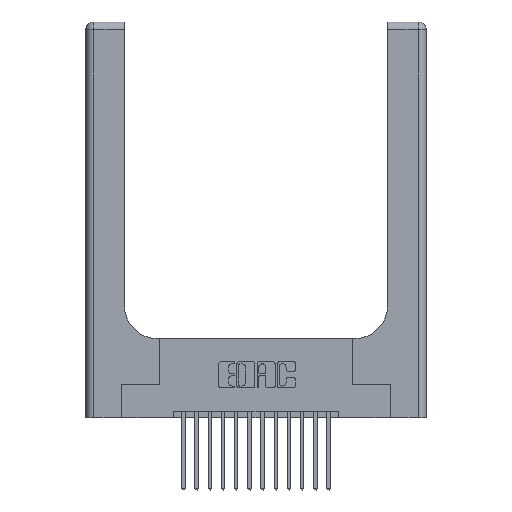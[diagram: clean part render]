
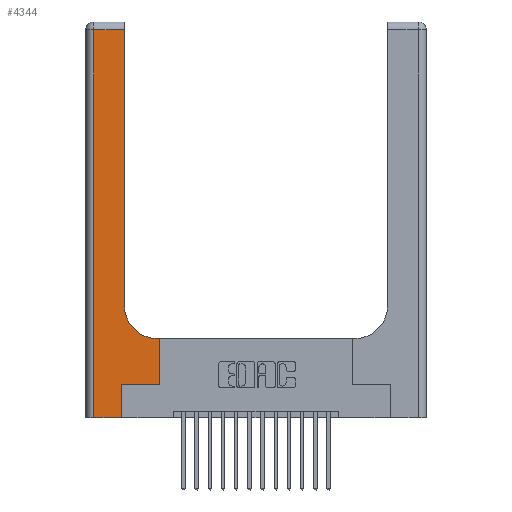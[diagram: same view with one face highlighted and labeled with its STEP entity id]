
A CAD part, top view. The second image highlights one B-rep face of the part: STEP entity #4344.
In plain terms, the highlighted planar face has unit normal (0, 0, 1).
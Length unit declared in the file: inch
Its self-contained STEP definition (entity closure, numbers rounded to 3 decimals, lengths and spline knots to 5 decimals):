
#13 = VECTOR ( 'NONE', #11765, 39.37008 ) ;
#380 = VECTOR ( 'NONE', #10703, 39.37008 ) ;
#407 = AXIS2_PLACEMENT_3D ( 'NONE', #4838, #15004, #6327 ) ;
#597 = LINE ( 'NONE', #6414, #7862 ) ;
#671 = LINE ( 'NONE', #1080, #4039 ) ;
#938 = VECTOR ( 'NONE', #16329, 39.37008 ) ;
#1080 = CARTESIAN_POINT ( 'NONE',  ( 0.269, 0.25, 0.37 ) ) ;
#1119 = CARTESIAN_POINT ( 'NONE',  ( 0.2915, 0.85, 0.37 ) ) ;
#1162 = ORIENTED_EDGE ( 'NONE', *, *, #1350, .T. ) ;
#1229 = VERTEX_POINT ( 'NONE', #1533 ) ;
#1254 = ORIENTED_EDGE ( 'NONE', *, *, #16557, .T. ) ;
#1350 = EDGE_CURVE ( 'NONE', #1229, #7404, #18650, .T. ) ;
#1461 = DIRECTION ( 'NONE',  ( -1., 0., 0. ) ) ;
#1533 = CARTESIAN_POINT ( 'NONE',  ( 0.5415, 0.6, 0.37 ) ) ;
#2022 = EDGE_CURVE ( 'NONE', #10979, #4656, #597, .T. ) ;
#2251 = VECTOR ( 'NONE', #11056, 39.37008 ) ;
#2411 = CARTESIAN_POINT ( 'NONE',  ( 0.06, 2.94, 0.37 ) ) ;
#2652 = AXIS2_PLACEMENT_3D ( 'NONE', #6569, #6552, #6879 ) ;
#2978 = EDGE_LOOP ( 'NONE', ( #9357, #15954, #17317, #1254, #3291, #14676, #6632, #12477, #1162 ) ) ;
#3042 = CARTESIAN_POINT ( 'NONE',  ( 0., 0., 0.37 ) ) ;
#3291 = ORIENTED_EDGE ( 'NONE', *, *, #2022, .T. ) ;
#3384 = LINE ( 'NONE', #3042, #13 ) ;
#3390 = PLANE ( 'NONE',  #407 ) ;
#4039 = VECTOR ( 'NONE', #11238, 39.37008 ) ;
#4344 = ADVANCED_FACE ( 'NONE', ( #7776 ), #3390, .F. ) ;
#4435 = LINE ( 'NONE', #15876, #15110 ) ;
#4656 = VERTEX_POINT ( 'NONE', #17050 ) ;
#4753 = LINE ( 'NONE', #6211, #938 ) ;
#4784 = EDGE_CURVE ( 'NONE', #7404, #6162, #4753, .T. ) ;
#4836 = CARTESIAN_POINT ( 'NONE',  ( 0.5585, 0.25, 0.37 ) ) ;
#4838 = CARTESIAN_POINT ( 'NONE',  ( 0., 3., 0.37 ) ) ;
#6162 = VERTEX_POINT ( 'NONE', #13524 ) ;
#6211 = CARTESIAN_POINT ( 'NONE',  ( 0.2915, 3., 0.37 ) ) ;
#6327 = DIRECTION ( 'NONE',  ( -1., 0., 0. ) ) ;
#6414 = CARTESIAN_POINT ( 'NONE',  ( 0.269, 0., 0.37 ) ) ;
#6552 = DIRECTION ( 'NONE',  ( 0., 0., -1. ) ) ;
#6569 = CARTESIAN_POINT ( 'NONE',  ( 0.5415, 0.85, 0.37 ) ) ;
#6632 = ORIENTED_EDGE ( 'NONE', *, *, #16886, .T. ) ;
#6784 = EDGE_CURVE ( 'NONE', #4656, #17263, #671, .T. ) ;
#6879 = DIRECTION ( 'NONE',  ( 1., 0., 0. ) ) ;
#7404 = VERTEX_POINT ( 'NONE', #1119 ) ;
#7583 = EDGE_CURVE ( 'NONE', #6162, #12037, #10626, .T. ) ;
#7776 = FACE_OUTER_BOUND ( 'NONE', #2978, .T. ) ;
#7862 = VECTOR ( 'NONE', #7889, 39.37008 ) ;
#7889 = DIRECTION ( 'NONE',  ( 0., 1., 0. ) ) ;
#8342 = VERTEX_POINT ( 'NONE', #8743 ) ;
#8743 = CARTESIAN_POINT ( 'NONE',  ( 0.06, 0., 0.37 ) ) ;
#8788 = CARTESIAN_POINT ( 'NONE',  ( 0.5585, 0.6, 0.37 ) ) ;
#9357 = ORIENTED_EDGE ( 'NONE', *, *, #4784, .T. ) ;
#9596 = CARTESIAN_POINT ( 'NONE',  ( 0.5585, 0.25, 0.37 ) ) ;
#10319 = VERTEX_POINT ( 'NONE', #8788 ) ;
#10626 = LINE ( 'NONE', #12674, #14455 ) ;
#10703 = DIRECTION ( 'NONE',  ( 0., -1., 0. ) ) ;
#10979 = VERTEX_POINT ( 'NONE', #11358 ) ;
#11056 = DIRECTION ( 'NONE',  ( 0., 1., 0. ) ) ;
#11238 = DIRECTION ( 'NONE',  ( 1., 0., 0. ) ) ;
#11358 = CARTESIAN_POINT ( 'NONE',  ( 0.269, 0., 0.37 ) ) ;
#11765 = DIRECTION ( 'NONE',  ( 1., 0., 0. ) ) ;
#12037 = VERTEX_POINT ( 'NONE', #2411 ) ;
#12477 = ORIENTED_EDGE ( 'NONE', *, *, #18569, .T. ) ;
#12674 = CARTESIAN_POINT ( 'NONE',  ( 0., 2.94, 0.37 ) ) ;
#12932 = EDGE_CURVE ( 'NONE', #12037, #8342, #15314, .T. ) ;
#13524 = CARTESIAN_POINT ( 'NONE',  ( 0.2915, 2.94, 0.37 ) ) ;
#13817 = LINE ( 'NONE', #9596, #2251 ) ;
#14102 = DIRECTION ( 'NONE',  ( -1., 0., 0. ) ) ;
#14455 = VECTOR ( 'NONE', #14102, 39.37008 ) ;
#14676 = ORIENTED_EDGE ( 'NONE', *, *, #6784, .T. ) ;
#15004 = DIRECTION ( 'NONE',  ( 0., 0., -1. ) ) ;
#15110 = VECTOR ( 'NONE', #1461, 39.37008 ) ;
#15314 = LINE ( 'NONE', #16187, #380 ) ;
#15876 = CARTESIAN_POINT ( 'NONE',  ( 0.2915, 0.6, 0.37 ) ) ;
#15954 = ORIENTED_EDGE ( 'NONE', *, *, #7583, .T. ) ;
#16187 = CARTESIAN_POINT ( 'NONE',  ( 0.06, 3., 0.37 ) ) ;
#16329 = DIRECTION ( 'NONE',  ( 0., 1., 0. ) ) ;
#16557 = EDGE_CURVE ( 'NONE', #8342, #10979, #3384, .T. ) ;
#16886 = EDGE_CURVE ( 'NONE', #17263, #10319, #13817, .T. ) ;
#17050 = CARTESIAN_POINT ( 'NONE',  ( 0.269, 0.25, 0.37 ) ) ;
#17263 = VERTEX_POINT ( 'NONE', #4836 ) ;
#17317 = ORIENTED_EDGE ( 'NONE', *, *, #12932, .T. ) ;
#18569 = EDGE_CURVE ( 'NONE', #10319, #1229, #4435, .T. ) ;
#18650 = CIRCLE ( 'NONE', #2652, 0.25 ) ;
